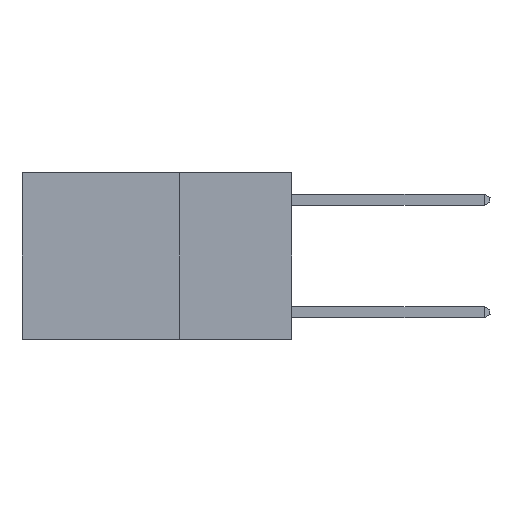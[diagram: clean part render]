
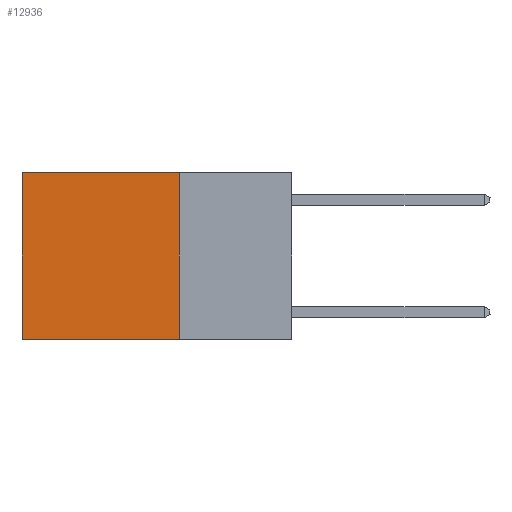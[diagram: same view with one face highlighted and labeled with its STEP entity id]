
A CAD part, left-side view. The second image highlights one B-rep face of the part: STEP entity #12936.
In plain terms, the highlighted planar face has unit normal (-1, 0, 0).
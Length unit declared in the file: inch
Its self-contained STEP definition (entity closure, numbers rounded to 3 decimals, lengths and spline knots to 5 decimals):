
#636 = EDGE_CURVE ( 'NONE', #10382, #2999, #5837, .T. ) ;
#2019 = VECTOR ( 'NONE', #9384, 39.37008 ) ;
#2356 = EDGE_LOOP ( 'NONE', ( #8891, #12517, #11245, #7100 ) ) ;
#2498 = CARTESIAN_POINT ( 'NONE',  ( 0.2625, 0.6, 0. ) ) ;
#2802 = VECTOR ( 'NONE', #7109, 39.37008 ) ;
#2999 = VERTEX_POINT ( 'NONE', #7092 ) ;
#3593 = LINE ( 'NONE', #2498, #11346 ) ;
#3656 = DIRECTION ( 'NONE',  ( 0., 0., -1. ) ) ;
#4424 = EDGE_CURVE ( 'NONE', #12442, #10136, #13166, .T. ) ;
#4454 = DIRECTION ( 'NONE',  ( 1., 0., 0. ) ) ;
#5614 = DIRECTION ( 'NONE',  ( 0., 0., -1. ) ) ;
#5812 = CARTESIAN_POINT ( 'NONE',  ( 0.2625, 0.6, 0. ) ) ;
#5837 = LINE ( 'NONE', #6306, #2019 ) ;
#5957 = CARTESIAN_POINT ( 'NONE',  ( 0.2625, 0.25, -0.37 ) ) ;
#6070 = DIRECTION ( 'NONE',  ( 0., 0., -1. ) ) ;
#6306 = CARTESIAN_POINT ( 'NONE',  ( 0.2625, 0.25, -0.37 ) ) ;
#6494 = PLANE ( 'NONE',  #9827 ) ;
#7092 = CARTESIAN_POINT ( 'NONE',  ( 0.2625, 0.6, -0.37 ) ) ;
#7100 = ORIENTED_EDGE ( 'NONE', *, *, #4424, .T. ) ;
#7109 = DIRECTION ( 'NONE',  ( 0., 1., 0. ) ) ;
#7476 = VECTOR ( 'NONE', #6070, 39.37008 ) ;
#8891 = ORIENTED_EDGE ( 'NONE', *, *, #11965, .T. ) ;
#9217 = LINE ( 'NONE', #13280, #7476 ) ;
#9384 = DIRECTION ( 'NONE',  ( 0., 1., 0. ) ) ;
#9520 = CARTESIAN_POINT ( 'NONE',  ( 0.2625, 0.25, 0. ) ) ;
#9642 = FACE_OUTER_BOUND ( 'NONE', #2356, .T. ) ;
#9827 = AXIS2_PLACEMENT_3D ( 'NONE', #11608, #4454, #5614 ) ;
#10136 = VERTEX_POINT ( 'NONE', #5812 ) ;
#10382 = VERTEX_POINT ( 'NONE', #5957 ) ;
#10727 = EDGE_CURVE ( 'NONE', #12442, #10382, #9217, .T. ) ;
#11245 = ORIENTED_EDGE ( 'NONE', *, *, #10727, .F. ) ;
#11346 = VECTOR ( 'NONE', #3656, 39.37008 ) ;
#11608 = CARTESIAN_POINT ( 'NONE',  ( 0.2625, 0.25, 0. ) ) ;
#11965 = EDGE_CURVE ( 'NONE', #10136, #2999, #3593, .T. ) ;
#12294 = CARTESIAN_POINT ( 'NONE',  ( 0.2625, 0.25, 0. ) ) ;
#12442 = VERTEX_POINT ( 'NONE', #9520 ) ;
#12517 = ORIENTED_EDGE ( 'NONE', *, *, #636, .F. ) ;
#12936 = ADVANCED_FACE ( 'NONE', ( #9642 ), #6494, .F. ) ;
#13166 = LINE ( 'NONE', #12294, #2802 ) ;
#13280 = CARTESIAN_POINT ( 'NONE',  ( 0.2625, 0.25, 0. ) ) ;
